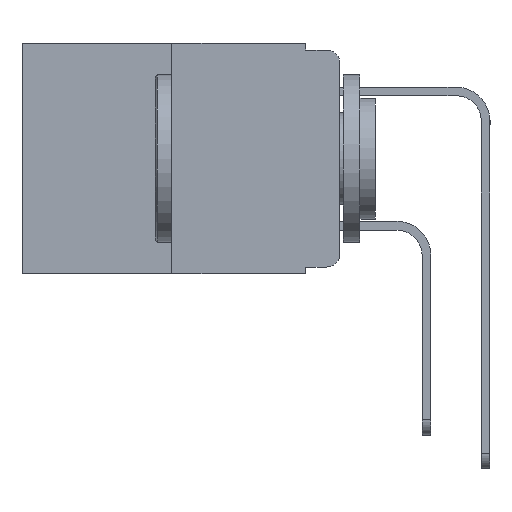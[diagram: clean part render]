
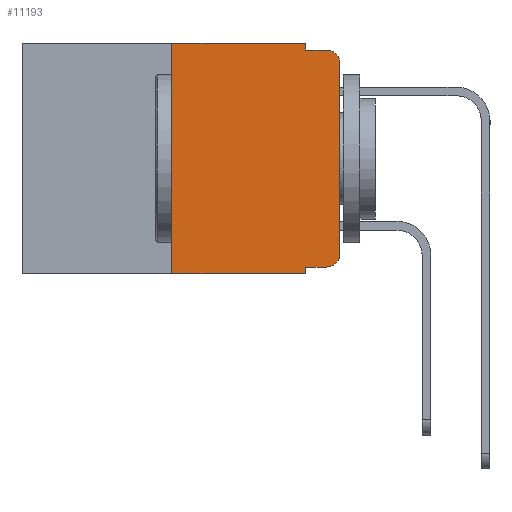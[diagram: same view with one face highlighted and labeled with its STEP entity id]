
A CAD part, left-side view. The second image highlights one B-rep face of the part: STEP entity #11193.
In plain terms, the highlighted planar face has unit normal (-1, 0, 0).
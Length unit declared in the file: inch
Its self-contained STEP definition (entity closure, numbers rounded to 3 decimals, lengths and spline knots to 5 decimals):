
#60 = CARTESIAN_POINT ( 'NONE',  ( 0., 0.051, 0. ) ) ;
#178 = ORIENTED_EDGE ( 'NONE', *, *, #16073, .T. ) ;
#1040 = CARTESIAN_POINT ( 'NONE',  ( 0., 0.473, -0.343 ) ) ;
#1222 = ORIENTED_EDGE ( 'NONE', *, *, #12072, .F. ) ;
#1243 = LINE ( 'NONE', #9956, #1735 ) ;
#1355 = DIRECTION ( 'NONE',  ( 0., 0., -1. ) ) ;
#1615 = DIRECTION ( 'NONE',  ( 0., 0., 1. ) ) ;
#1711 = ORIENTED_EDGE ( 'NONE', *, *, #3325, .F. ) ;
#1735 = VECTOR ( 'NONE', #2288, 39.37008 ) ;
#1885 = CARTESIAN_POINT ( 'NONE',  ( 0., 0., -0.03 ) ) ;
#2016 = LINE ( 'NONE', #18198, #13681 ) ;
#2248 = DIRECTION ( 'NONE',  ( 1., 0., 0. ) ) ;
#2288 = DIRECTION ( 'NONE',  ( 0., 0., -1. ) ) ;
#2652 = DIRECTION ( 'NONE',  ( 0., -1., 0. ) ) ;
#2906 = VERTEX_POINT ( 'NONE', #1885 ) ;
#3164 = CARTESIAN_POINT ( 'NONE',  ( 0., 0.02, -0.01 ) ) ;
#3325 = EDGE_CURVE ( 'NONE', #3857, #4357, #2016, .T. ) ;
#3485 = VECTOR ( 'NONE', #12670, 39.37008 ) ;
#3632 = VECTOR ( 'NONE', #3664, 39.37008 ) ;
#3664 = DIRECTION ( 'NONE',  ( 0., -1., 0. ) ) ;
#3857 = VERTEX_POINT ( 'NONE', #17504 ) ;
#4357 = VERTEX_POINT ( 'NONE', #60 ) ;
#4921 = ORIENTED_EDGE ( 'NONE', *, *, #13078, .F. ) ;
#5434 = VERTEX_POINT ( 'NONE', #6175 ) ;
#5533 = CARTESIAN_POINT ( 'NONE',  ( 0., 0.02, -0.03 ) ) ;
#5682 = ORIENTED_EDGE ( 'NONE', *, *, #8037, .T. ) ;
#5835 = CARTESIAN_POINT ( 'NONE',  ( 0., 0.051, -0.01 ) ) ;
#5977 = CIRCLE ( 'NONE', #17661, 0.02 ) ;
#6091 = AXIS2_PLACEMENT_3D ( 'NONE', #18762, #2248, #12920 ) ;
#6108 = VERTEX_POINT ( 'NONE', #6849 ) ;
#6149 = ORIENTED_EDGE ( 'NONE', *, *, #7028, .T. ) ;
#6175 = CARTESIAN_POINT ( 'NONE',  ( 0., 0.02, -0.333 ) ) ;
#6276 = EDGE_CURVE ( 'NONE', #6108, #19424, #19036, .T. ) ;
#6364 = ORIENTED_EDGE ( 'NONE', *, *, #10083, .F. ) ;
#6836 = ORIENTED_EDGE ( 'NONE', *, *, #9028, .F. ) ;
#6849 = CARTESIAN_POINT ( 'NONE',  ( 0., 0.25, -0.343 ) ) ;
#7028 = EDGE_CURVE ( 'NONE', #5434, #11634, #5977, .T. ) ;
#7053 = DIRECTION ( 'NONE',  ( 0., 0., -1. ) ) ;
#7710 = LINE ( 'NONE', #9744, #3632 ) ;
#7899 = EDGE_LOOP ( 'NONE', ( #178, #16443, #4921, #1222, #1711, #6364, #14335, #6836, #5682, #6149 ) ) ;
#8014 = VECTOR ( 'NONE', #16875, 39.37008 ) ;
#8037 = EDGE_CURVE ( 'NONE', #10043, #5434, #18966, .T. ) ;
#9028 = EDGE_CURVE ( 'NONE', #10043, #19424, #1243, .T. ) ;
#9161 = VECTOR ( 'NONE', #13372, 39.37008 ) ;
#9339 = CARTESIAN_POINT ( 'NONE',  ( 0., 0., -0.313 ) ) ;
#9648 = LINE ( 'NONE', #10396, #9161 ) ;
#9744 = CARTESIAN_POINT ( 'NONE',  ( 0., 0.051, -0.01 ) ) ;
#9956 = CARTESIAN_POINT ( 'NONE',  ( 0., 0.051, 0. ) ) ;
#10043 = VERTEX_POINT ( 'NONE', #13677 ) ;
#10077 = FACE_OUTER_BOUND ( 'NONE', #7899, .T. ) ;
#10083 = EDGE_CURVE ( 'NONE', #6108, #3857, #10814, .T. ) ;
#10396 = CARTESIAN_POINT ( 'NONE',  ( 0., 0.051, 0. ) ) ;
#10587 = DIRECTION ( 'NONE',  ( -1., 0., 0. ) ) ;
#10716 = VECTOR ( 'NONE', #2652, 39.37008 ) ;
#10814 = LINE ( 'NONE', #12266, #14301 ) ;
#10900 = CARTESIAN_POINT ( 'NONE',  ( 0., 0., 0. ) ) ;
#10942 = VERTEX_POINT ( 'NONE', #3164 ) ;
#11162 = CARTESIAN_POINT ( 'NONE',  ( 0., 0.051, -0.333 ) ) ;
#11193 = ADVANCED_FACE ( 'NONE', ( #10077 ), #14270, .F. ) ;
#11634 = VERTEX_POINT ( 'NONE', #9339 ) ;
#12072 = EDGE_CURVE ( 'NONE', #4357, #19287, #9648, .T. ) ;
#12266 = CARTESIAN_POINT ( 'NONE',  ( 0., 0.25, 0. ) ) ;
#12670 = DIRECTION ( 'NONE',  ( 0., -1., 0. ) ) ;
#12920 = DIRECTION ( 'NONE',  ( 0., 0., -1. ) ) ;
#13078 = EDGE_CURVE ( 'NONE', #19287, #10942, #7710, .T. ) ;
#13372 = DIRECTION ( 'NONE',  ( 0., 0., -1. ) ) ;
#13677 = CARTESIAN_POINT ( 'NONE',  ( 0., 0.051, -0.333 ) ) ;
#13681 = VECTOR ( 'NONE', #18284, 39.37008 ) ;
#14270 = PLANE ( 'NONE',  #6091 ) ;
#14301 = VECTOR ( 'NONE', #1615, 39.37008 ) ;
#14335 = ORIENTED_EDGE ( 'NONE', *, *, #6276, .T. ) ;
#15072 = EDGE_CURVE ( 'NONE', #2906, #10942, #17121, .T. ) ;
#15391 = CARTESIAN_POINT ( 'NONE',  ( 0., 0.051, -0.343 ) ) ;
#15508 = LINE ( 'NONE', #10900, #8014 ) ;
#16032 = DIRECTION ( 'NONE',  ( -1., 0., 0. ) ) ;
#16073 = EDGE_CURVE ( 'NONE', #11634, #2906, #15508, .T. ) ;
#16443 = ORIENTED_EDGE ( 'NONE', *, *, #15072, .T. ) ;
#16875 = DIRECTION ( 'NONE',  ( 0., 0., 1. ) ) ;
#17121 = CIRCLE ( 'NONE', #17253, 0.02 ) ;
#17253 = AXIS2_PLACEMENT_3D ( 'NONE', #5533, #16032, #7053 ) ;
#17504 = CARTESIAN_POINT ( 'NONE',  ( 0., 0.25, 0. ) ) ;
#17661 = AXIS2_PLACEMENT_3D ( 'NONE', #19407, #10587, #1355 ) ;
#18198 = CARTESIAN_POINT ( 'NONE',  ( 0., 0.473, 0. ) ) ;
#18284 = DIRECTION ( 'NONE',  ( 0., -1., 0. ) ) ;
#18762 = CARTESIAN_POINT ( 'NONE',  ( 0., 0.473, 0. ) ) ;
#18966 = LINE ( 'NONE', #11162, #3485 ) ;
#19036 = LINE ( 'NONE', #1040, #10716 ) ;
#19287 = VERTEX_POINT ( 'NONE', #5835 ) ;
#19407 = CARTESIAN_POINT ( 'NONE',  ( 0., 0.02, -0.313 ) ) ;
#19424 = VERTEX_POINT ( 'NONE', #15391 ) ;
